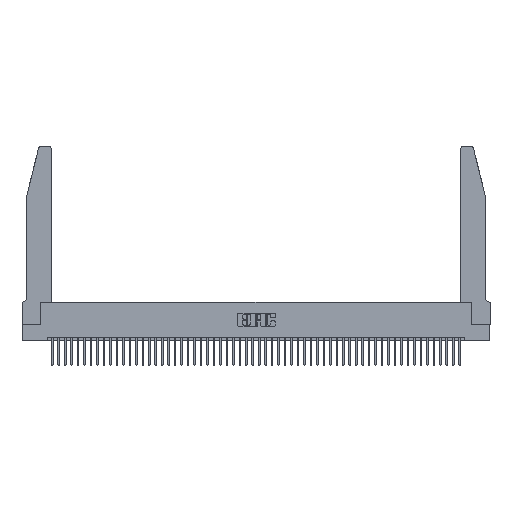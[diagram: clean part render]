
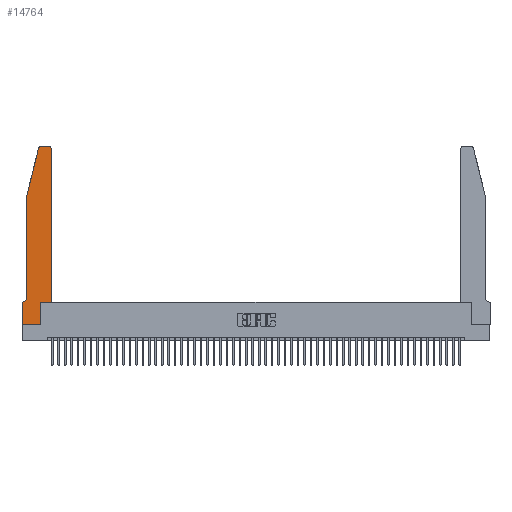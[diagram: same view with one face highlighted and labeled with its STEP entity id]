
A CAD part, top view. The second image highlights one B-rep face of the part: STEP entity #14764.
In plain terms, the highlighted planar face has unit normal (0, 0, 1).
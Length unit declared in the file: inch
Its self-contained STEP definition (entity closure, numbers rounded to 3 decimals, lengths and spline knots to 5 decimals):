
#386 = EDGE_CURVE ( 'NONE', #26215, #23217, #39629, .T. ) ;
#416 = DIRECTION ( 'NONE',  ( -1., 0., 0. ) ) ;
#531 = VECTOR ( 'NONE', #31126, 39.37008 ) ;
#709 = DIRECTION ( 'NONE',  ( 1., 0., 0. ) ) ;
#1534 = VERTEX_POINT ( 'NONE', #51799 ) ;
#1560 = CARTESIAN_POINT ( 'NONE',  ( 0.0755, 2., 0.37 ) ) ;
#1749 = EDGE_CURVE ( 'NONE', #17168, #6337, #51340, .T. ) ;
#2670 = CARTESIAN_POINT ( 'NONE',  ( 0., 0., 0.37 ) ) ;
#2833 = EDGE_CURVE ( 'NONE', #21671, #32219, #46223, .T. ) ;
#4411 = VECTOR ( 'NONE', #416, 39.37008 ) ;
#5784 = FACE_OUTER_BOUND ( 'NONE', #13625, .T. ) ;
#6140 = PLANE ( 'NONE',  #23609 ) ;
#6337 = VERTEX_POINT ( 'NONE', #51715 ) ;
#6683 = VERTEX_POINT ( 'NONE', #9846 ) ;
#7190 = CIRCLE ( 'NONE', #33224, 0.03 ) ;
#7641 = VECTOR ( 'NONE', #44392, 39.37008 ) ;
#8089 = VECTOR ( 'NONE', #11044, 39.37008 ) ;
#8953 = DIRECTION ( 'NONE',  ( 0., 0., -1. ) ) ;
#9846 = CARTESIAN_POINT ( 'NONE',  ( 0., 0., 0.37 ) ) ;
#11044 = DIRECTION ( 'NONE',  ( 0., -1., 0. ) ) ;
#11314 = ORIENTED_EDGE ( 'NONE', *, *, #16435, .T. ) ;
#11385 = LINE ( 'NONE', #46986, #531 ) ;
#12453 = ORIENTED_EDGE ( 'NONE', *, *, #386, .T. ) ;
#13347 = VECTOR ( 'NONE', #18151, 39.37008 ) ;
#13625 = EDGE_LOOP ( 'NONE', ( #19115, #32071, #12453, #28642, #24315, #11314, #22861, #25752, #42489, #49692, #30171, #32259 ) ) ;
#14004 = VERTEX_POINT ( 'NONE', #33988 ) ;
#14332 = DIRECTION ( 'NONE',  ( 1., 0., 0. ) ) ;
#14611 = VECTOR ( 'NONE', #30849, 39.37008 ) ;
#14764 = ADVANCED_FACE ( 'NONE', ( #5784 ), #6140, .T. ) ;
#15210 = LINE ( 'NONE', #20685, #4411 ) ;
#15445 = EDGE_CURVE ( 'NONE', #6683, #40382, #45245, .T. ) ;
#15587 = EDGE_CURVE ( 'NONE', #16008, #17168, #49570, .T. ) ;
#15788 = CARTESIAN_POINT ( 'NONE',  ( 0.0055, 0.35, 0.37 ) ) ;
#16008 = VERTEX_POINT ( 'NONE', #30290 ) ;
#16435 = EDGE_CURVE ( 'NONE', #32219, #27128, #15210, .T. ) ;
#17168 = VERTEX_POINT ( 'NONE', #20796 ) ;
#18151 = DIRECTION ( 'NONE',  ( 1., 0., 0. ) ) ;
#18857 = LINE ( 'NONE', #23020, #8089 ) ;
#19115 = ORIENTED_EDGE ( 'NONE', *, *, #1749, .T. ) ;
#19441 = LINE ( 'NONE', #29394, #49993 ) ;
#19703 = DIRECTION ( 'NONE',  ( 0., 0., 1. ) ) ;
#19851 = EDGE_CURVE ( 'NONE', #1534, #16008, #42795, .T. ) ;
#20355 = VECTOR ( 'NONE', #23515, 39.37008 ) ;
#20685 = CARTESIAN_POINT ( 'NONE',  ( 0.0755, 0.35, 0.37 ) ) ;
#20710 = EDGE_CURVE ( 'NONE', #14004, #1534, #24012, .T. ) ;
#20796 = CARTESIAN_POINT ( 'NONE',  ( 0.4205, 2.75, 0.37 ) ) ;
#21085 = CARTESIAN_POINT ( 'NONE',  ( 0.2605, 2.75, 0.37 ) ) ;
#21375 = AXIS2_PLACEMENT_3D ( 'NONE', #33000, #8953, #37038 ) ;
#21671 = VERTEX_POINT ( 'NONE', #31833 ) ;
#22804 = EDGE_CURVE ( 'NONE', #23217, #21671, #18857, .T. ) ;
#22861 = ORIENTED_EDGE ( 'NONE', *, *, #30850, .T. ) ;
#23020 = CARTESIAN_POINT ( 'NONE',  ( 0.0755, 2., 0.37 ) ) ;
#23062 = CARTESIAN_POINT ( 'NONE',  ( 0., 0.35, 0.37 ) ) ;
#23217 = VERTEX_POINT ( 'NONE', #1560 ) ;
#23515 = DIRECTION ( 'NONE',  ( 0., 1., 0. ) ) ;
#23609 = AXIS2_PLACEMENT_3D ( 'NONE', #34269, #38266, #14332 ) ;
#24012 = LINE ( 'NONE', #49876, #13347 ) ;
#24315 = ORIENTED_EDGE ( 'NONE', *, *, #2833, .T. ) ;
#24987 = DIRECTION ( 'NONE',  ( 0., 0., 1. ) ) ;
#25107 = DIRECTION ( 'NONE',  ( -1., 0., 0. ) ) ;
#25752 = ORIENTED_EDGE ( 'NONE', *, *, #15445, .T. ) ;
#26215 = VERTEX_POINT ( 'NONE', #39067 ) ;
#27128 = VERTEX_POINT ( 'NONE', #23062 ) ;
#27537 = CARTESIAN_POINT ( 'NONE',  ( 0.4505, 0.35, 0.37 ) ) ;
#28642 = ORIENTED_EDGE ( 'NONE', *, *, #22804, .T. ) ;
#29394 = CARTESIAN_POINT ( 'NONE',  ( 0.2865, 0.35, 0.37 ) ) ;
#30171 = ORIENTED_EDGE ( 'NONE', *, *, #19851, .T. ) ;
#30290 = CARTESIAN_POINT ( 'NONE',  ( 0.4505, 2.72, 0.37 ) ) ;
#30849 = DIRECTION ( 'NONE',  ( 1., 0., 0. ) ) ;
#30850 = EDGE_CURVE ( 'NONE', #27128, #6683, #11385, .T. ) ;
#31126 = DIRECTION ( 'NONE',  ( 0., -1., 0. ) ) ;
#31833 = CARTESIAN_POINT ( 'NONE',  ( 0.0755, 0.42, 0.37 ) ) ;
#32071 = ORIENTED_EDGE ( 'NONE', *, *, #36472, .T. ) ;
#32219 = VERTEX_POINT ( 'NONE', #15788 ) ;
#32259 = ORIENTED_EDGE ( 'NONE', *, *, #15587, .T. ) ;
#32306 = AXIS2_PLACEMENT_3D ( 'NONE', #43597, #19703, #47594 ) ;
#33000 = CARTESIAN_POINT ( 'NONE',  ( 0.0055, 0.42, 0.37 ) ) ;
#33224 = AXIS2_PLACEMENT_3D ( 'NONE', #48840, #24987, #709 ) ;
#33404 = DIRECTION ( 'NONE',  ( 0., 1., 0. ) ) ;
#33988 = CARTESIAN_POINT ( 'NONE',  ( 0.2865, 0.35, 0.37 ) ) ;
#34269 = CARTESIAN_POINT ( 'NONE',  ( 0., 0.35, 0.37 ) ) ;
#36472 = EDGE_CURVE ( 'NONE', #6337, #26215, #7190, .T. ) ;
#37038 = DIRECTION ( 'NONE',  ( -1., 0., 0. ) ) ;
#38266 = DIRECTION ( 'NONE',  ( 0., 0., 1. ) ) ;
#39067 = CARTESIAN_POINT ( 'NONE',  ( 0.25487, 2.72718, 0.37 ) ) ;
#39629 = LINE ( 'NONE', #40372, #7641 ) ;
#40372 = CARTESIAN_POINT ( 'NONE',  ( 0.0755, 2., 0.37 ) ) ;
#40382 = VERTEX_POINT ( 'NONE', #42637 ) ;
#40736 = VECTOR ( 'NONE', #25107, 39.37008 ) ;
#42489 = ORIENTED_EDGE ( 'NONE', *, *, #43143, .T. ) ;
#42637 = CARTESIAN_POINT ( 'NONE',  ( 0.2865, 0., 0.37 ) ) ;
#42795 = LINE ( 'NONE', #27537, #20355 ) ;
#43143 = EDGE_CURVE ( 'NONE', #40382, #14004, #19441, .T. ) ;
#43597 = CARTESIAN_POINT ( 'NONE',  ( 0.4205, 2.72, 0.37 ) ) ;
#44392 = DIRECTION ( 'NONE',  ( -0.239, -0.971, 0. ) ) ;
#45245 = LINE ( 'NONE', #2670, #14611 ) ;
#46223 = CIRCLE ( 'NONE', #21375, 0.07 ) ;
#46986 = CARTESIAN_POINT ( 'NONE',  ( 0., 0., 0.37 ) ) ;
#47594 = DIRECTION ( 'NONE',  ( 1., 0., 0. ) ) ;
#48840 = CARTESIAN_POINT ( 'NONE',  ( 0.284, 2.72, 0.37 ) ) ;
#49570 = CIRCLE ( 'NONE', #32306, 0.03 ) ;
#49692 = ORIENTED_EDGE ( 'NONE', *, *, #20710, .T. ) ;
#49876 = CARTESIAN_POINT ( 'NONE',  ( 0.4505, 0.35, 0.37 ) ) ;
#49993 = VECTOR ( 'NONE', #33404, 39.37008 ) ;
#51340 = LINE ( 'NONE', #21085, #40736 ) ;
#51715 = CARTESIAN_POINT ( 'NONE',  ( 0.284, 2.75, 0.37 ) ) ;
#51799 = CARTESIAN_POINT ( 'NONE',  ( 0.4505, 0.35, 0.37 ) ) ;
